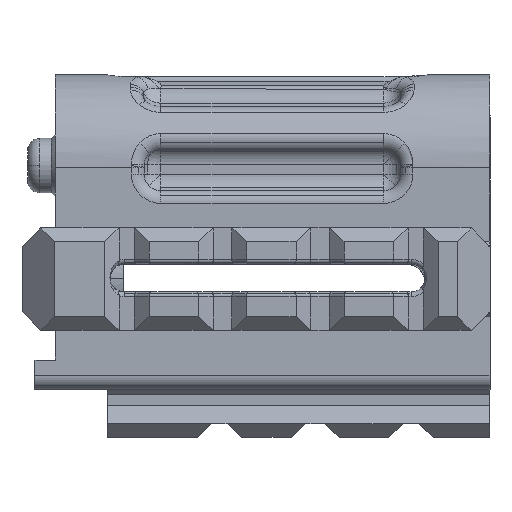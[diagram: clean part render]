
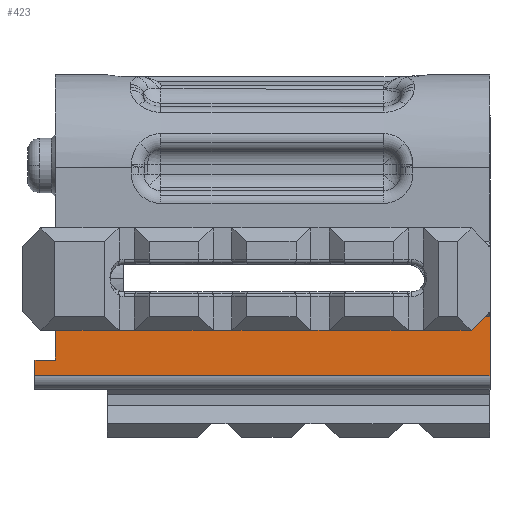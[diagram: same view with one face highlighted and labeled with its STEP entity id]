
A CAD part, top view. The second image highlights one B-rep face of the part: STEP entity #423.
In plain terms, the highlighted planar face has unit normal (0, 0, 1).
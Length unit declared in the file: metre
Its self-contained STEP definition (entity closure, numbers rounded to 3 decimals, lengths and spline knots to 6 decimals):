
#423=ADVANCED_FACE('0:341',(#1256),#1257,.T.);
#1256=FACE_OUTER_BOUND('',#2247,.T.);
#1257=PLANE('',#2248);
#2247=EDGE_LOOP('',(#5504,#5505,#5506,#5507,#5508,#5509));
#2248=AXIS2_PLACEMENT_3D('',#5510,#5511,#5512);
#5504=ORIENTED_EDGE('',*,*,#7626,.F.);
#5505=ORIENTED_EDGE('',*,*,#7627,.T.);
#5506=ORIENTED_EDGE('',*,*,#7464,.T.);
#5507=ORIENTED_EDGE('',*,*,#7409,.T.);
#5508=ORIENTED_EDGE('',*,*,#7625,.F.);
#5509=ORIENTED_EDGE('',*,*,#7628,.T.);
#5510=CARTESIAN_POINT('',(0.0127,0.08261,0.0201));
#5511=DIRECTION('',(0.0,0.,1.0));
#5512=DIRECTION('',(0.0,-1.0,0.));
#7409=EDGE_CURVE('0:2675',#9231,#9229,#9232,.T.);
#7464=EDGE_CURVE('0:3320',#9307,#9231,#9311,.T.);
#7625=EDGE_CURVE('0:3227',#9529,#9229,#9531,.T.);
#7626=EDGE_CURVE('0:3311',#9532,#9533,#9534,.T.);
#7627=EDGE_CURVE('0:3317',#9532,#9307,#9535,.T.);
#7628=EDGE_CURVE('0:3323',#9529,#9533,#9536,.T.);
#9229=VERTEX_POINT('',#13967);
#9231=VERTEX_POINT('',#13969);
#9232=LINE('',#13970,#13971);
#9307=VERTEX_POINT('',#14241);
#9311=LINE('',#14247,#14248);
#9529=VERTEX_POINT('',#14714);
#9531=LINE('',#14716,#14717);
#9532=VERTEX_POINT('',#14718);
#9533=VERTEX_POINT('',#14719);
#9534=LINE('',#14720,#14721);
#9535=LINE('',#14722,#14723);
#9536=LINE('',#14724,#14725);
#13967=CARTESIAN_POINT('',(0.0083,0.00306,0.0201));
#13969=CARTESIAN_POINT('',(0.0083,0.00641,0.0201));
#13970=CARTESIAN_POINT('',(0.0083,0.045001,0.0201));
#13971=VECTOR('',#17351,0.00335);
#14241=CARTESIAN_POINT('',(0.0127,0.00641,0.0201));
#14247=CARTESIAN_POINT('',(0.0127,0.00641,0.0201));
#14248=VECTOR('',#17443,0.0044);
#14714=CARTESIAN_POINT('',(0.106318,0.00306,0.0201));
#14716=CARTESIAN_POINT('',(0.0127,0.00306,0.0201));
#14717=VECTOR('',#17686,0.098018);
#14718=CARTESIAN_POINT('',(0.0127,0.015707,0.0201));
#14719=CARTESIAN_POINT('',(0.106318,0.015707,0.0201));
#14720=CARTESIAN_POINT('',(0.009702,0.015707,0.0201));
#14721=VECTOR('',#17687,0.093618);
#14722=CARTESIAN_POINT('',(0.0127,0.060786,0.0201));
#14723=VECTOR('',#17688,0.009297);
#14724=CARTESIAN_POINT('',(0.106318,0.071272,0.0201));
#14725=VECTOR('',#17689,0.012647);
#17351=DIRECTION('',(0.0,-1.0,0.));
#17443=DIRECTION('',(-1.0,0.0,0.0));
#17686=DIRECTION('',(-1.0,0.0,0.0));
#17687=DIRECTION('',(1.0,0.0,0.0));
#17688=DIRECTION('',(0.0,-1.0,0.));
#17689=DIRECTION('',(0.0,1.0,0.));
